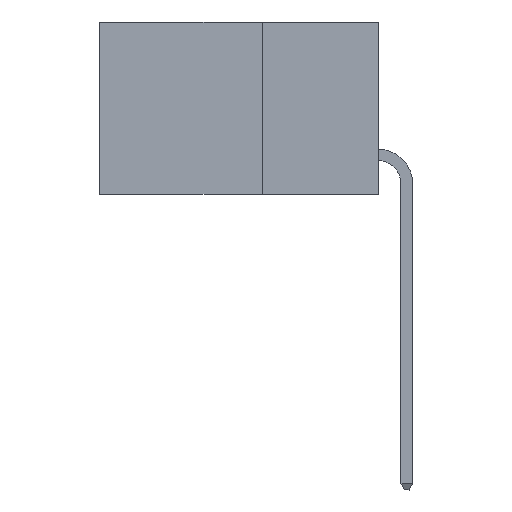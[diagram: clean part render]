
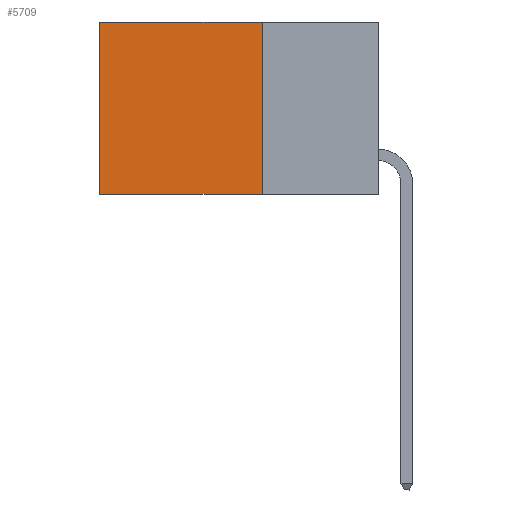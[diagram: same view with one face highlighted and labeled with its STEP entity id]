
A CAD part, left-side view. The second image highlights one B-rep face of the part: STEP entity #5709.
In plain terms, the highlighted planar face has unit normal (-1, 0, 0).
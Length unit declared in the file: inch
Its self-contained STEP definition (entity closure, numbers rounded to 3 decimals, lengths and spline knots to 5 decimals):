
#740 = VERTEX_POINT ( 'NONE', #31284 ) ;
#2548 = LINE ( 'NONE', #6658, #11434 ) ;
#3144 = CARTESIAN_POINT ( 'NONE',  ( 0.298, 0.25, 0. ) ) ;
#3912 = CARTESIAN_POINT ( 'NONE',  ( 0.298, 0.25, -0.37 ) ) ;
#5677 = VERTEX_POINT ( 'NONE', #24530 ) ;
#5709 = ADVANCED_FACE ( 'NONE', ( #7406 ), #5894, .F. ) ;
#5894 = PLANE ( 'NONE',  #13479 ) ;
#6485 = LINE ( 'NONE', #15983, #21105 ) ;
#6658 = CARTESIAN_POINT ( 'NONE',  ( 0.298, 0.6, 0. ) ) ;
#7052 = EDGE_CURVE ( 'NONE', #5677, #18928, #12718, .T. ) ;
#7406 = FACE_OUTER_BOUND ( 'NONE', #20956, .T. ) ;
#7977 = ORIENTED_EDGE ( 'NONE', *, *, #14279, .F. ) ;
#7983 = DIRECTION ( 'NONE',  ( 0., 0., -1. ) ) ;
#8992 = ORIENTED_EDGE ( 'NONE', *, *, #7052, .F. ) ;
#9682 = DIRECTION ( 'NONE',  ( 1., 0., 0. ) ) ;
#10592 = DIRECTION ( 'NONE',  ( 0., 1., 0. ) ) ;
#11434 = VECTOR ( 'NONE', #28734, 39.37008 ) ;
#12718 = LINE ( 'NONE', #3144, #21119 ) ;
#13479 = AXIS2_PLACEMENT_3D ( 'NONE', #21925, #9682, #17214 ) ;
#14279 = EDGE_CURVE ( 'NONE', #18928, #15655, #6485, .T. ) ;
#15655 = VERTEX_POINT ( 'NONE', #28677 ) ;
#15983 = CARTESIAN_POINT ( 'NONE',  ( 0.298, 0.25, -0.37 ) ) ;
#17214 = DIRECTION ( 'NONE',  ( 0., 0., -1. ) ) ;
#18928 = VERTEX_POINT ( 'NONE', #3912 ) ;
#20164 = CARTESIAN_POINT ( 'NONE',  ( 0.298, 0.25, 0. ) ) ;
#20956 = EDGE_LOOP ( 'NONE', ( #28798, #7977, #8992, #22240 ) ) ;
#21105 = VECTOR ( 'NONE', #21125, 39.37008 ) ;
#21119 = VECTOR ( 'NONE', #7983, 39.37008 ) ;
#21125 = DIRECTION ( 'NONE',  ( 0., 1., 0. ) ) ;
#21925 = CARTESIAN_POINT ( 'NONE',  ( 0.298, 0.25, 0. ) ) ;
#22240 = ORIENTED_EDGE ( 'NONE', *, *, #26464, .T. ) ;
#23563 = EDGE_CURVE ( 'NONE', #740, #15655, #2548, .T. ) ;
#23955 = VECTOR ( 'NONE', #10592, 39.37008 ) ;
#24530 = CARTESIAN_POINT ( 'NONE',  ( 0.298, 0.25, 0. ) ) ;
#26464 = EDGE_CURVE ( 'NONE', #5677, #740, #27410, .T. ) ;
#27410 = LINE ( 'NONE', #20164, #23955 ) ;
#28677 = CARTESIAN_POINT ( 'NONE',  ( 0.298, 0.6, -0.37 ) ) ;
#28734 = DIRECTION ( 'NONE',  ( 0., 0., -1. ) ) ;
#28798 = ORIENTED_EDGE ( 'NONE', *, *, #23563, .T. ) ;
#31284 = CARTESIAN_POINT ( 'NONE',  ( 0.298, 0.6, 0. ) ) ;
